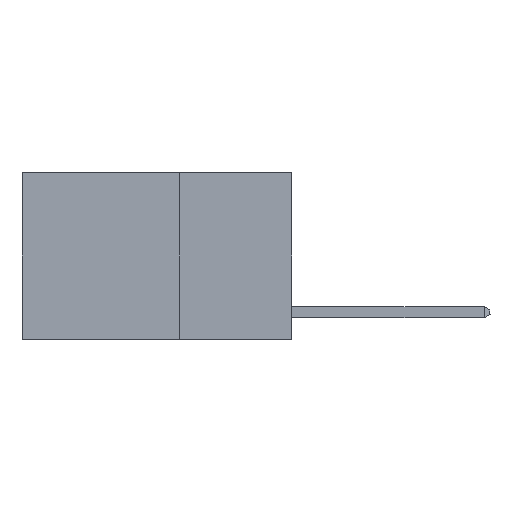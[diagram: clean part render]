
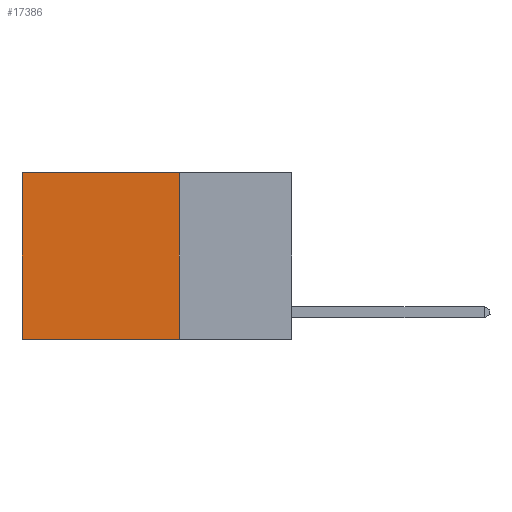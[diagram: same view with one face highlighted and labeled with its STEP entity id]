
A CAD part, left-side view. The second image highlights one B-rep face of the part: STEP entity #17386.
In plain terms, the highlighted planar face has unit normal (-1, 0, 0).
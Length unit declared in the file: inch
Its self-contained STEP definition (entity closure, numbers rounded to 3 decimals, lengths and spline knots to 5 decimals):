
#190 = VERTEX_POINT ( 'NONE', #6666 ) ;
#2004 = ORIENTED_EDGE ( 'NONE', *, *, #8302, .T. ) ;
#2319 = CARTESIAN_POINT ( 'NONE',  ( 0.2625, 0.25, 0. ) ) ;
#3838 = DIRECTION ( 'NONE',  ( 1., 0., 0. ) ) ;
#4576 = CARTESIAN_POINT ( 'NONE',  ( 0.2625, 0.25, 0. ) ) ;
#4608 = EDGE_LOOP ( 'NONE', ( #12745, #15181, #18981, #2004 ) ) ;
#5651 = VECTOR ( 'NONE', #18817, 39.37008 ) ;
#6666 = CARTESIAN_POINT ( 'NONE',  ( 0.2625, 0.6, -0.37 ) ) ;
#6721 = CARTESIAN_POINT ( 'NONE',  ( 0.2625, 0.25, 0. ) ) ;
#6818 = VERTEX_POINT ( 'NONE', #7953 ) ;
#7284 = VERTEX_POINT ( 'NONE', #4576 ) ;
#7953 = CARTESIAN_POINT ( 'NONE',  ( 0.2625, 0.25, -0.37 ) ) ;
#8302 = EDGE_CURVE ( 'NONE', #7284, #17883, #14327, .T. ) ;
#9826 = CARTESIAN_POINT ( 'NONE',  ( 0.2625, 0.25, -0.37 ) ) ;
#10045 = EDGE_CURVE ( 'NONE', #17883, #190, #10267, .T. ) ;
#10267 = LINE ( 'NONE', #12411, #17279 ) ;
#11332 = PLANE ( 'NONE',  #14008 ) ;
#11911 = FACE_OUTER_BOUND ( 'NONE', #4608, .T. ) ;
#12411 = CARTESIAN_POINT ( 'NONE',  ( 0.2625, 0.6, 0. ) ) ;
#12745 = ORIENTED_EDGE ( 'NONE', *, *, #10045, .T. ) ;
#13155 = DIRECTION ( 'NONE',  ( 0., 0., -1. ) ) ;
#13831 = VECTOR ( 'NONE', #17182, 39.37008 ) ;
#14008 = AXIS2_PLACEMENT_3D ( 'NONE', #2319, #3838, #14352 ) ;
#14200 = CARTESIAN_POINT ( 'NONE',  ( 0.2625, 0.6, 0. ) ) ;
#14327 = LINE ( 'NONE', #6721, #13831 ) ;
#14352 = DIRECTION ( 'NONE',  ( 0., 0., -1. ) ) ;
#14789 = VECTOR ( 'NONE', #13155, 39.37008 ) ;
#15043 = EDGE_CURVE ( 'NONE', #6818, #190, #17604, .T. ) ;
#15181 = ORIENTED_EDGE ( 'NONE', *, *, #15043, .F. ) ;
#15212 = EDGE_CURVE ( 'NONE', #7284, #6818, #18795, .T. ) ;
#16164 = CARTESIAN_POINT ( 'NONE',  ( 0.2625, 0.25, 0. ) ) ;
#16920 = DIRECTION ( 'NONE',  ( 0., 0., -1. ) ) ;
#17182 = DIRECTION ( 'NONE',  ( 0., 1., 0. ) ) ;
#17279 = VECTOR ( 'NONE', #16920, 39.37008 ) ;
#17386 = ADVANCED_FACE ( 'NONE', ( #11911 ), #11332, .F. ) ;
#17604 = LINE ( 'NONE', #9826, #5651 ) ;
#17883 = VERTEX_POINT ( 'NONE', #14200 ) ;
#18795 = LINE ( 'NONE', #16164, #14789 ) ;
#18817 = DIRECTION ( 'NONE',  ( 0., 1., 0. ) ) ;
#18981 = ORIENTED_EDGE ( 'NONE', *, *, #15212, .F. ) ;
